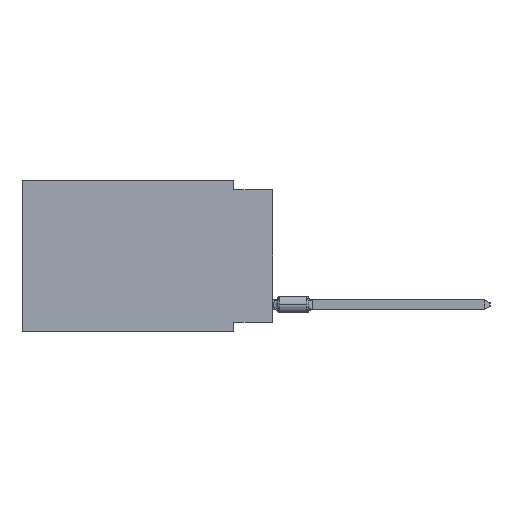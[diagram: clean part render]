
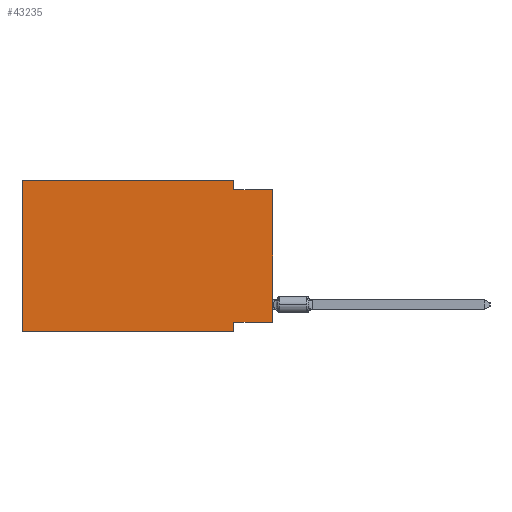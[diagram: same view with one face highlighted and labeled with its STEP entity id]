
A CAD part, left-side view. The second image highlights one B-rep face of the part: STEP entity #43235.
In plain terms, the highlighted planar face has unit normal (-1, 0, 0).
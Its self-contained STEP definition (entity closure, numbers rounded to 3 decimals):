
#66 = ORIENTED_EDGE ( 'NONE', *, *, #79212, .F. ) ;
#1596 = ORIENTED_EDGE ( 'NONE', *, *, #28624, .F. ) ;
#5636 = VECTOR ( 'NONE', #66071, 1000. ) ;
#6063 = DIRECTION ( 'NONE',  ( 0., 0., -1. ) ) ;
#7270 = EDGE_CURVE ( 'NONE', #81329, #45999, #39355, .T. ) ;
#10968 = CARTESIAN_POINT ( 'NONE',  ( 0., 2.54, -0.635 ) ) ;
#12234 = CARTESIAN_POINT ( 'NONE',  ( 0., 16.383, 0. ) ) ;
#15143 = LINE ( 'NONE', #41885, #19759 ) ;
#18454 = CARTESIAN_POINT ( 'NONE',  ( 0., 0., -0.635 ) ) ;
#19476 = CARTESIAN_POINT ( 'NONE',  ( 0., 0., 0. ) ) ;
#19759 = VECTOR ( 'NONE', #75684, 1000. ) ;
#21710 = VECTOR ( 'NONE', #48456, 1000. ) ;
#23578 = CARTESIAN_POINT ( 'NONE',  ( 0., 0., -0.635 ) ) ;
#25036 = LINE ( 'NONE', #18454, #33648 ) ;
#25096 = VERTEX_POINT ( 'NONE', #55282 ) ;
#26950 = DIRECTION ( 'NONE',  ( 0., -1., 0. ) ) ;
#28624 = EDGE_CURVE ( 'NONE', #43108, #64868, #25036, .T. ) ;
#29086 = CARTESIAN_POINT ( 'NONE',  ( 0., 16.383, 0. ) ) ;
#30630 = ORIENTED_EDGE ( 'NONE', *, *, #70417, .T. ) ;
#31405 = ORIENTED_EDGE ( 'NONE', *, *, #77523, .F. ) ;
#32659 = LINE ( 'NONE', #60283, #85846 ) ;
#33648 = VECTOR ( 'NONE', #45210, 1000. ) ;
#34438 = LINE ( 'NONE', #40572, #21710 ) ;
#37059 = AXIS2_PLACEMENT_3D ( 'NONE', #12234, #80207, #6063 ) ;
#37397 = CARTESIAN_POINT ( 'NONE',  ( 0., 2.54, 0. ) ) ;
#39290 = CARTESIAN_POINT ( 'NONE',  ( 0., 2.54, -9.906 ) ) ;
#39355 = LINE ( 'NONE', #79708, #67792 ) ;
#40572 = CARTESIAN_POINT ( 'NONE',  ( 0., 16.383, 0. ) ) ;
#40586 = LINE ( 'NONE', #39290, #5636 ) ;
#41348 = EDGE_CURVE ( 'NONE', #81012, #25096, #32659, .T. ) ;
#41885 = CARTESIAN_POINT ( 'NONE',  ( 0., 2.54, 0. ) ) ;
#43108 = VERTEX_POINT ( 'NONE', #10968 ) ;
#43235 = ADVANCED_FACE ( 'NONE', ( #60913 ), #60478, .F. ) ;
#44627 = EDGE_LOOP ( 'NONE', ( #30630, #1596, #66, #68298, #31405, #69891, #72614, #76900 ) ) ;
#45210 = DIRECTION ( 'NONE',  ( 0., -1., 0. ) ) ;
#45977 = LINE ( 'NONE', #74477, #50358 ) ;
#45999 = VERTEX_POINT ( 'NONE', #59065 ) ;
#48456 = DIRECTION ( 'NONE',  ( 0., -1., 0. ) ) ;
#50358 = VECTOR ( 'NONE', #72744, 1000. ) ;
#55282 = CARTESIAN_POINT ( 'NONE',  ( 0., 2.54, -9.906 ) ) ;
#56719 = VERTEX_POINT ( 'NONE', #29086 ) ;
#59033 = VERTEX_POINT ( 'NONE', #37397 ) ;
#59065 = CARTESIAN_POINT ( 'NONE',  ( 0., 2.54, -9.271 ) ) ;
#59844 = DIRECTION ( 'NONE',  ( 0., 0., 1. ) ) ;
#60283 = CARTESIAN_POINT ( 'NONE',  ( 0., 16.383, -9.906 ) ) ;
#60478 = PLANE ( 'NONE',  #37059 ) ;
#60913 = FACE_OUTER_BOUND ( 'NONE', #44627, .T. ) ;
#62122 = VECTOR ( 'NONE', #59844, 1000. ) ;
#64868 = VERTEX_POINT ( 'NONE', #23578 ) ;
#66071 = DIRECTION ( 'NONE',  ( 0., 0., -1. ) ) ;
#67792 = VECTOR ( 'NONE', #78860, 1000. ) ;
#68298 = ORIENTED_EDGE ( 'NONE', *, *, #72405, .F. ) ;
#69891 = ORIENTED_EDGE ( 'NONE', *, *, #41348, .T. ) ;
#70417 = EDGE_CURVE ( 'NONE', #81329, #64868, #74728, .T. ) ;
#72405 = EDGE_CURVE ( 'NONE', #56719, #59033, #34438, .T. ) ;
#72614 = ORIENTED_EDGE ( 'NONE', *, *, #77911, .F. ) ;
#72744 = DIRECTION ( 'NONE',  ( 0., 0., 1. ) ) ;
#74477 = CARTESIAN_POINT ( 'NONE',  ( 0., 16.383, 0. ) ) ;
#74728 = LINE ( 'NONE', #19476, #62122 ) ;
#75684 = DIRECTION ( 'NONE',  ( 0., 0., -1. ) ) ;
#76900 = ORIENTED_EDGE ( 'NONE', *, *, #7270, .F. ) ;
#77523 = EDGE_CURVE ( 'NONE', #81012, #56719, #45977, .T. ) ;
#77911 = EDGE_CURVE ( 'NONE', #45999, #25096, #40586, .T. ) ;
#77934 = CARTESIAN_POINT ( 'NONE',  ( 0., 0., -9.271 ) ) ;
#78860 = DIRECTION ( 'NONE',  ( 0., 1., 0. ) ) ;
#79212 = EDGE_CURVE ( 'NONE', #59033, #43108, #15143, .T. ) ;
#79708 = CARTESIAN_POINT ( 'NONE',  ( 0., 0., -9.271 ) ) ;
#80207 = DIRECTION ( 'NONE',  ( 1., 0., 0. ) ) ;
#81012 = VERTEX_POINT ( 'NONE', #84595 ) ;
#81329 = VERTEX_POINT ( 'NONE', #77934 ) ;
#84595 = CARTESIAN_POINT ( 'NONE',  ( 0., 16.383, -9.906 ) ) ;
#85846 = VECTOR ( 'NONE', #26950, 1000. ) ;
